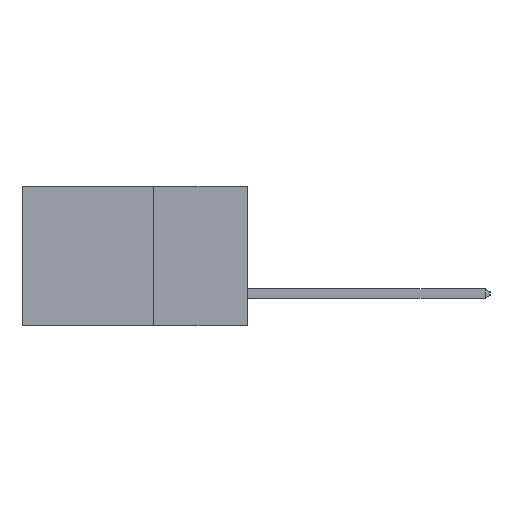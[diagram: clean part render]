
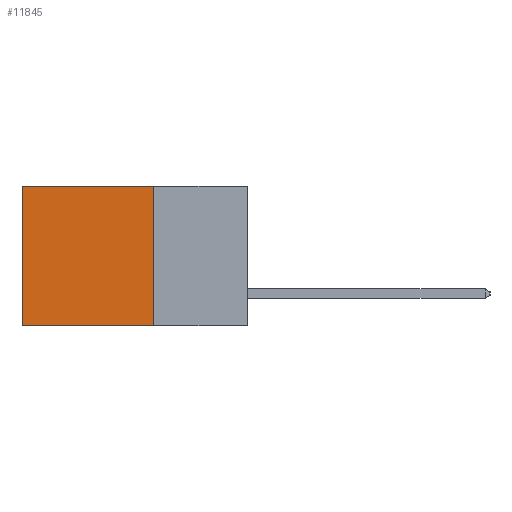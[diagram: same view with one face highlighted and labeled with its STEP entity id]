
A CAD part, left-side view. The second image highlights one B-rep face of the part: STEP entity #11845.
In plain terms, the highlighted planar face has unit normal (-1, 0, 0).
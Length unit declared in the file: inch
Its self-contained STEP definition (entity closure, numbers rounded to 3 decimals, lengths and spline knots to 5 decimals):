
#548 = ORIENTED_EDGE ( 'NONE', *, *, #8917, .F. ) ;
#1848 = LINE ( 'NONE', #17573, #6504 ) ;
#2132 = CARTESIAN_POINT ( 'NONE',  ( 0.298, 0.6, 0. ) ) ;
#2211 = CARTESIAN_POINT ( 'NONE',  ( 0.298, 0.25, -0.37 ) ) ;
#2947 = VERTEX_POINT ( 'NONE', #2211 ) ;
#3477 = DIRECTION ( 'NONE',  ( 0., 0., -1. ) ) ;
#6046 = DIRECTION ( 'NONE',  ( 0., 0., -1. ) ) ;
#6504 = VECTOR ( 'NONE', #7545, 39.37008 ) ;
#6648 = ORIENTED_EDGE ( 'NONE', *, *, #16380, .T. ) ;
#7195 = LINE ( 'NONE', #12054, #21249 ) ;
#7545 = DIRECTION ( 'NONE',  ( 0., 1., 0. ) ) ;
#7960 = PLANE ( 'NONE',  #21326 ) ;
#8587 = VECTOR ( 'NONE', #20730, 39.37008 ) ;
#8917 = EDGE_CURVE ( 'NONE', #2947, #15504, #24468, .T. ) ;
#9281 = FACE_OUTER_BOUND ( 'NONE', #24213, .T. ) ;
#9403 = VERTEX_POINT ( 'NONE', #2132 ) ;
#11697 = EDGE_CURVE ( 'NONE', #20599, #9403, #1848, .T. ) ;
#11750 = ORIENTED_EDGE ( 'NONE', *, *, #11697, .T. ) ;
#11845 = ADVANCED_FACE ( 'NONE', ( #9281 ), #7960, .F. ) ;
#11965 = DIRECTION ( 'NONE',  ( 0., 0., -1. ) ) ;
#12054 = CARTESIAN_POINT ( 'NONE',  ( 0.298, 0.25, 0. ) ) ;
#13072 = ORIENTED_EDGE ( 'NONE', *, *, #21710, .F. ) ;
#15440 = CARTESIAN_POINT ( 'NONE',  ( 0.298, 0.6, 0. ) ) ;
#15504 = VERTEX_POINT ( 'NONE', #16798 ) ;
#16077 = CARTESIAN_POINT ( 'NONE',  ( 0.298, 0.25, 0. ) ) ;
#16380 = EDGE_CURVE ( 'NONE', #9403, #15504, #22717, .T. ) ;
#16798 = CARTESIAN_POINT ( 'NONE',  ( 0.298, 0.6, -0.37 ) ) ;
#17527 = VECTOR ( 'NONE', #3477, 39.37008 ) ;
#17573 = CARTESIAN_POINT ( 'NONE',  ( 0.298, 0.25, 0. ) ) ;
#18077 = DIRECTION ( 'NONE',  ( 1., 0., 0. ) ) ;
#18761 = CARTESIAN_POINT ( 'NONE',  ( 0.298, 0.25, -0.37 ) ) ;
#20599 = VERTEX_POINT ( 'NONE', #24594 ) ;
#20730 = DIRECTION ( 'NONE',  ( 0., 1., 0. ) ) ;
#21249 = VECTOR ( 'NONE', #11965, 39.37008 ) ;
#21326 = AXIS2_PLACEMENT_3D ( 'NONE', #16077, #18077, #6046 ) ;
#21710 = EDGE_CURVE ( 'NONE', #20599, #2947, #7195, .T. ) ;
#22717 = LINE ( 'NONE', #15440, #17527 ) ;
#24213 = EDGE_LOOP ( 'NONE', ( #6648, #548, #13072, #11750 ) ) ;
#24468 = LINE ( 'NONE', #18761, #8587 ) ;
#24594 = CARTESIAN_POINT ( 'NONE',  ( 0.298, 0.25, 0. ) ) ;
